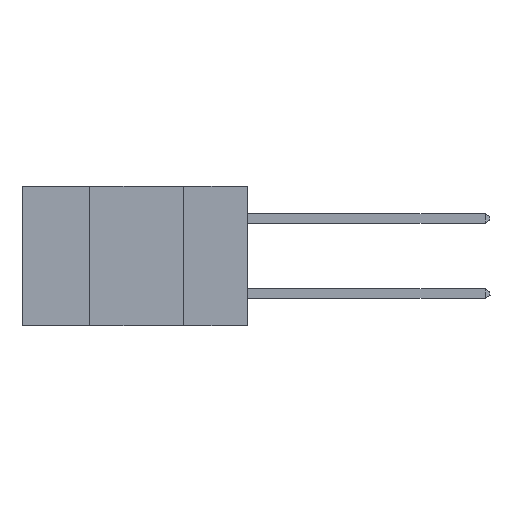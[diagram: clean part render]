
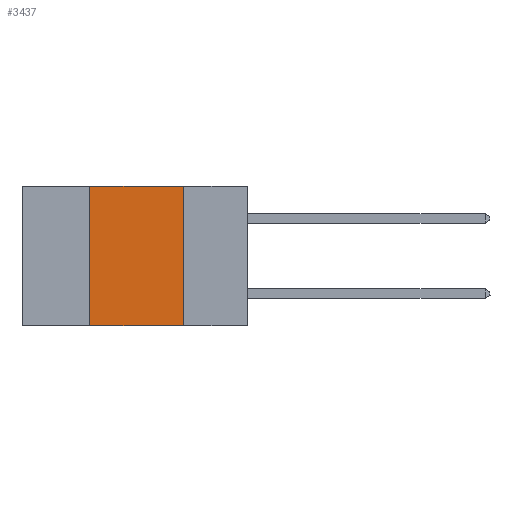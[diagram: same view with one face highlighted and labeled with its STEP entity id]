
A CAD part, left-side view. The second image highlights one B-rep face of the part: STEP entity #3437.
In plain terms, the highlighted planar face has unit normal (-1, 0, 0).
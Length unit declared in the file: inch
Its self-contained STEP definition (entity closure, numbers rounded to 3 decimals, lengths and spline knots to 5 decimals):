
#31 = LINE ( 'NONE', #13381, #14338 ) ;
#97 = VECTOR ( 'NONE', #14325, 39.37008 ) ;
#1575 = EDGE_CURVE ( 'NONE', #9664, #14225, #1886, .T. ) ;
#1886 = LINE ( 'NONE', #16473, #97 ) ;
#1891 = CARTESIAN_POINT ( 'NONE',  ( 0., 0.17, 0. ) ) ;
#2296 = AXIS2_PLACEMENT_3D ( 'NONE', #13142, #11853, #4133 ) ;
#2524 = EDGE_LOOP ( 'NONE', ( #10270, #14357, #3584, #10620 ) ) ;
#2615 = VERTEX_POINT ( 'NONE', #10276 ) ;
#3090 = EDGE_CURVE ( 'NONE', #13970, #2615, #31, .T. ) ;
#3437 = ADVANCED_FACE ( 'NONE', ( #4966 ), #10511, .F. ) ;
#3584 = ORIENTED_EDGE ( 'NONE', *, *, #13377, .F. ) ;
#4133 = DIRECTION ( 'NONE',  ( 0., 0., -1. ) ) ;
#4966 = FACE_OUTER_BOUND ( 'NONE', #2524, .T. ) ;
#6094 = CARTESIAN_POINT ( 'NONE',  ( 0., 0.17, -0.37 ) ) ;
#6343 = EDGE_CURVE ( 'NONE', #2615, #14225, #15246, .T. ) ;
#7419 = VECTOR ( 'NONE', #14078, 39.37008 ) ;
#8837 = LINE ( 'NONE', #10461, #7419 ) ;
#9664 = VERTEX_POINT ( 'NONE', #9840 ) ;
#9840 = CARTESIAN_POINT ( 'NONE',  ( 0., 0.42, -0.37 ) ) ;
#10270 = ORIENTED_EDGE ( 'NONE', *, *, #6343, .F. ) ;
#10276 = CARTESIAN_POINT ( 'NONE',  ( 0., 0.17, 0. ) ) ;
#10461 = CARTESIAN_POINT ( 'NONE',  ( 0., 0.42, 0. ) ) ;
#10511 = PLANE ( 'NONE',  #2296 ) ;
#10620 = ORIENTED_EDGE ( 'NONE', *, *, #1575, .T. ) ;
#10891 = DIRECTION ( 'NONE',  ( 0., -1., 0. ) ) ;
#11853 = DIRECTION ( 'NONE',  ( 1., 0., 0. ) ) ;
#12829 = VECTOR ( 'NONE', #13389, 39.37008 ) ;
#13142 = CARTESIAN_POINT ( 'NONE',  ( 0., 0.6, 0. ) ) ;
#13377 = EDGE_CURVE ( 'NONE', #9664, #13970, #8837, .T. ) ;
#13381 = CARTESIAN_POINT ( 'NONE',  ( 0., 0.6, 0. ) ) ;
#13389 = DIRECTION ( 'NONE',  ( 0., 0., -1. ) ) ;
#13970 = VERTEX_POINT ( 'NONE', #14758 ) ;
#14078 = DIRECTION ( 'NONE',  ( 0., 0., 1. ) ) ;
#14225 = VERTEX_POINT ( 'NONE', #6094 ) ;
#14325 = DIRECTION ( 'NONE',  ( 0., -1., 0. ) ) ;
#14338 = VECTOR ( 'NONE', #10891, 39.37008 ) ;
#14357 = ORIENTED_EDGE ( 'NONE', *, *, #3090, .F. ) ;
#14758 = CARTESIAN_POINT ( 'NONE',  ( 0., 0.42, 0. ) ) ;
#15246 = LINE ( 'NONE', #1891, #12829 ) ;
#16473 = CARTESIAN_POINT ( 'NONE',  ( 0., 0.6, -0.37 ) ) ;
